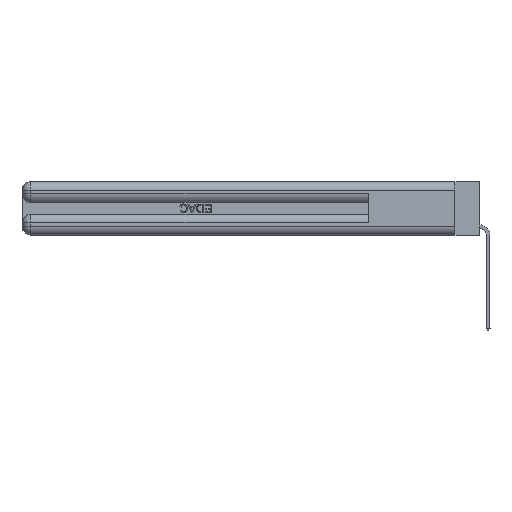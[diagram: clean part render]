
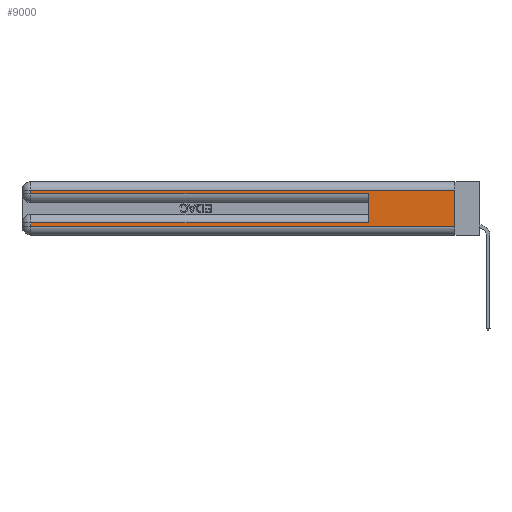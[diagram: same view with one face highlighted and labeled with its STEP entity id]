
A CAD part, left-side view. The second image highlights one B-rep face of the part: STEP entity #9000.
In plain terms, the highlighted planar face has unit normal (-1, 0, 0).
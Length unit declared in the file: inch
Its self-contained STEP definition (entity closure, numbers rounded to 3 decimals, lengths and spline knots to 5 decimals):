
#1063 = ORIENTED_EDGE ( 'NONE', *, *, #11987, .F. ) ;
#1898 = LINE ( 'NONE', #27159, #15914 ) ;
#1952 = CARTESIAN_POINT ( 'NONE',  ( 0., 0., 0.285 ) ) ;
#2655 = CARTESIAN_POINT ( 'NONE',  ( 0., 2.94, 0.285 ) ) ;
#3301 = LINE ( 'NONE', #11697, #9537 ) ;
#3592 = ORIENTED_EDGE ( 'NONE', *, *, #11782, .T. ) ;
#4563 = CARTESIAN_POINT ( 'NONE',  ( 0., 0., 0.37 ) ) ;
#4648 = DIRECTION ( 'NONE',  ( 0., -1., 0. ) ) ;
#4654 = CARTESIAN_POINT ( 'NONE',  ( 0., 0.6, 0.145 ) ) ;
#4822 = VECTOR ( 'NONE', #22958, 39.37008 ) ;
#4841 = ORIENTED_EDGE ( 'NONE', *, *, #7072, .T. ) ;
#5692 = VECTOR ( 'NONE', #4648, 39.37008 ) ;
#5981 = VERTEX_POINT ( 'NONE', #32855 ) ;
#6438 = EDGE_CURVE ( 'NONE', #11694, #22592, #3301, .T. ) ;
#6560 = CARTESIAN_POINT ( 'NONE',  ( 0., 0., 0.37 ) ) ;
#7072 = EDGE_CURVE ( 'NONE', #5981, #11694, #19289, .T. ) ;
#7282 = VERTEX_POINT ( 'NONE', #20532 ) ;
#9000 = ADVANCED_FACE ( 'NONE', ( #18104 ), #9241, .F. ) ;
#9241 = PLANE ( 'NONE',  #27175 ) ;
#9254 = CARTESIAN_POINT ( 'NONE',  ( 0., 0., 0.31 ) ) ;
#9537 = VECTOR ( 'NONE', #29876, 39.37008 ) ;
#9724 = LINE ( 'NONE', #26800, #21138 ) ;
#10261 = EDGE_CURVE ( 'NONE', #22592, #7282, #18820, .T. ) ;
#10717 = CARTESIAN_POINT ( 'NONE',  ( 0., 0., 0.085 ) ) ;
#10912 = CARTESIAN_POINT ( 'NONE',  ( 0., 2.94, 0.31 ) ) ;
#11023 = ORIENTED_EDGE ( 'NONE', *, *, #24312, .F. ) ;
#11072 = VERTEX_POINT ( 'NONE', #29225 ) ;
#11572 = DIRECTION ( 'NONE',  ( 0., -1., 0. ) ) ;
#11694 = VERTEX_POINT ( 'NONE', #10912 ) ;
#11697 = CARTESIAN_POINT ( 'NONE',  ( 0., 2.94, 0.37 ) ) ;
#11782 = EDGE_CURVE ( 'NONE', #14785, #17348, #1898, .T. ) ;
#11852 = DIRECTION ( 'NONE',  ( 0., 0., -1. ) ) ;
#11987 = EDGE_CURVE ( 'NONE', #27461, #7282, #30104, .T. ) ;
#13085 = DIRECTION ( 'NONE',  ( 0., 1., 0. ) ) ;
#14785 = VERTEX_POINT ( 'NONE', #24366 ) ;
#15121 = ORIENTED_EDGE ( 'NONE', *, *, #18984, .T. ) ;
#15123 = DIRECTION ( 'NONE',  ( 0., 0., -1. ) ) ;
#15914 = VECTOR ( 'NONE', #11572, 39.37008 ) ;
#16750 = ORIENTED_EDGE ( 'NONE', *, *, #24673, .T. ) ;
#17348 = VERTEX_POINT ( 'NONE', #17545 ) ;
#17545 = CARTESIAN_POINT ( 'NONE',  ( 0., 0., 0.06 ) ) ;
#18104 = FACE_OUTER_BOUND ( 'NONE', #24877, .T. ) ;
#18460 = VECTOR ( 'NONE', #30039, 39.37008 ) ;
#18820 = LINE ( 'NONE', #1952, #5692 ) ;
#18984 = EDGE_CURVE ( 'NONE', #27461, #11072, #20050, .T. ) ;
#19289 = LINE ( 'NONE', #9254, #18460 ) ;
#20050 = LINE ( 'NONE', #10717, #26130 ) ;
#20532 = CARTESIAN_POINT ( 'NONE',  ( 0., 0.6, 0.285 ) ) ;
#21138 = VECTOR ( 'NONE', #29387, 39.37008 ) ;
#22592 = VERTEX_POINT ( 'NONE', #2655 ) ;
#22958 = DIRECTION ( 'NONE',  ( 0., 0., 1. ) ) ;
#24312 = EDGE_CURVE ( 'NONE', #5981, #17348, #32504, .T. ) ;
#24366 = CARTESIAN_POINT ( 'NONE',  ( 0., 2.94, 0.06 ) ) ;
#24673 = EDGE_CURVE ( 'NONE', #11072, #14785, #9724, .T. ) ;
#24738 = DIRECTION ( 'NONE',  ( 1., 0., 0. ) ) ;
#24877 = EDGE_LOOP ( 'NONE', ( #11023, #4841, #32569, #26497, #1063, #15121, #16750, #3592 ) ) ;
#26130 = VECTOR ( 'NONE', #13085, 39.37008 ) ;
#26497 = ORIENTED_EDGE ( 'NONE', *, *, #10261, .T. ) ;
#26800 = CARTESIAN_POINT ( 'NONE',  ( 0., 2.94, 0.37 ) ) ;
#27159 = CARTESIAN_POINT ( 'NONE',  ( 0., 0., 0.06 ) ) ;
#27175 = AXIS2_PLACEMENT_3D ( 'NONE', #6560, #24738, #11852 ) ;
#27461 = VERTEX_POINT ( 'NONE', #32215 ) ;
#29225 = CARTESIAN_POINT ( 'NONE',  ( 0., 2.94, 0.085 ) ) ;
#29387 = DIRECTION ( 'NONE',  ( 0., 0., -1. ) ) ;
#29876 = DIRECTION ( 'NONE',  ( 0., 0., -1. ) ) ;
#30039 = DIRECTION ( 'NONE',  ( 0., 1., 0. ) ) ;
#30104 = LINE ( 'NONE', #4654, #4822 ) ;
#31680 = VECTOR ( 'NONE', #15123, 39.37008 ) ;
#32215 = CARTESIAN_POINT ( 'NONE',  ( 0., 0.6, 0.085 ) ) ;
#32504 = LINE ( 'NONE', #4563, #31680 ) ;
#32569 = ORIENTED_EDGE ( 'NONE', *, *, #6438, .T. ) ;
#32855 = CARTESIAN_POINT ( 'NONE',  ( 0., 0., 0.31 ) ) ;
